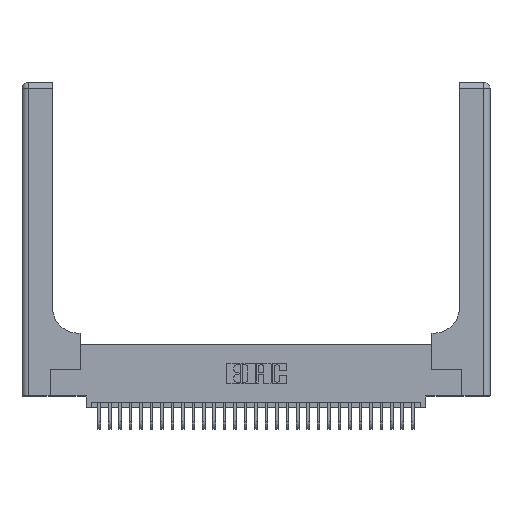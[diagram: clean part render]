
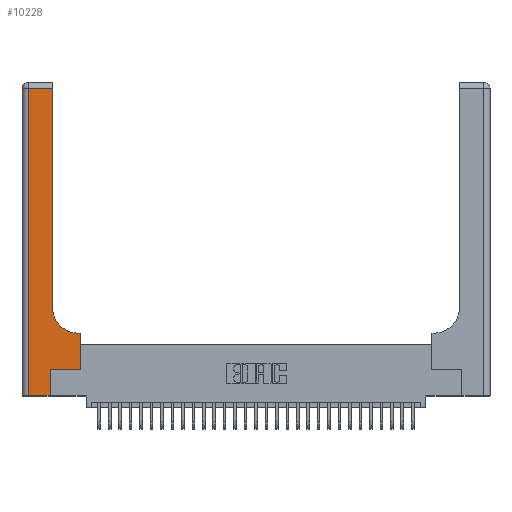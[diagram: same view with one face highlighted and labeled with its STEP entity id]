
A CAD part, top view. The second image highlights one B-rep face of the part: STEP entity #10228.
In plain terms, the highlighted planar face has unit normal (0, 0, 1).
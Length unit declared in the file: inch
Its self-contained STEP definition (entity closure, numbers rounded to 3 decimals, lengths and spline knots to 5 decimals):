
#24 = CARTESIAN_POINT ( 'NONE',  ( 0.2915, 0.85, 0.37 ) ) ;
#1550 = DIRECTION ( 'NONE',  ( 1., 0., 0. ) ) ;
#2169 = VECTOR ( 'NONE', #17892, 39.37008 ) ;
#2900 = LINE ( 'NONE', #7260, #30195 ) ;
#3365 = EDGE_LOOP ( 'NONE', ( #22565, #10003, #14203, #11431, #7960, #29017, #22181, #14543, #21084 ) ) ;
#5346 = EDGE_CURVE ( 'NONE', #19292, #30485, #27529, .T. ) ;
#5491 = CARTESIAN_POINT ( 'NONE',  ( 0.5585, 0.25, 0.37 ) ) ;
#5791 = VECTOR ( 'NONE', #11875, 39.37008 ) ;
#5969 = EDGE_CURVE ( 'NONE', #30485, #29714, #19609, .T. ) ;
#6583 = VERTEX_POINT ( 'NONE', #24 ) ;
#7260 = CARTESIAN_POINT ( 'NONE',  ( 0.269, 0., 0.37 ) ) ;
#7372 = LINE ( 'NONE', #30796, #19226 ) ;
#7460 = EDGE_CURVE ( 'NONE', #29104, #20316, #25124, .T. ) ;
#7960 = ORIENTED_EDGE ( 'NONE', *, *, #15478, .T. ) ;
#8972 = AXIS2_PLACEMENT_3D ( 'NONE', #14369, #19128, #1550 ) ;
#9488 = PLANE ( 'NONE',  #21902 ) ;
#9693 = DIRECTION ( 'NONE',  ( 0., 0., -1. ) ) ;
#9805 = CARTESIAN_POINT ( 'NONE',  ( 0., 3., 0.37 ) ) ;
#10003 = ORIENTED_EDGE ( 'NONE', *, *, #23485, .T. ) ;
#10132 = LINE ( 'NONE', #32572, #5791 ) ;
#10228 = ADVANCED_FACE ( 'NONE', ( #17512 ), #9488, .F. ) ;
#10370 = CARTESIAN_POINT ( 'NONE',  ( 0.5585, 0.25, 0.37 ) ) ;
#10698 = LINE ( 'NONE', #12680, #26083 ) ;
#11087 = CIRCLE ( 'NONE', #8972, 0.25 ) ;
#11431 = ORIENTED_EDGE ( 'NONE', *, *, #5969, .T. ) ;
#11765 = EDGE_CURVE ( 'NONE', #30705, #14472, #10698, .T. ) ;
#11875 = DIRECTION ( 'NONE',  ( 0., 1., 0. ) ) ;
#12680 = CARTESIAN_POINT ( 'NONE',  ( 0.2915, 0.6, 0.37 ) ) ;
#13956 = EDGE_CURVE ( 'NONE', #6583, #17723, #10132, .T. ) ;
#14203 = ORIENTED_EDGE ( 'NONE', *, *, #5346, .T. ) ;
#14369 = CARTESIAN_POINT ( 'NONE',  ( 0.5415, 0.85, 0.37 ) ) ;
#14432 = CARTESIAN_POINT ( 'NONE',  ( 0., 0., 0.37 ) ) ;
#14472 = VERTEX_POINT ( 'NONE', #17046 ) ;
#14543 = ORIENTED_EDGE ( 'NONE', *, *, #11765, .T. ) ;
#15191 = CARTESIAN_POINT ( 'NONE',  ( 0.06, 0., 0.37 ) ) ;
#15478 = EDGE_CURVE ( 'NONE', #29714, #29104, #2900, .T. ) ;
#16627 = CARTESIAN_POINT ( 'NONE',  ( 0.06, 2.94, 0.37 ) ) ;
#16750 = CARTESIAN_POINT ( 'NONE',  ( 0.269, 0.25, 0.37 ) ) ;
#17046 = CARTESIAN_POINT ( 'NONE',  ( 0.5415, 0.6, 0.37 ) ) ;
#17512 = FACE_OUTER_BOUND ( 'NONE', #3365, .T. ) ;
#17723 = VERTEX_POINT ( 'NONE', #25579 ) ;
#17892 = DIRECTION ( 'NONE',  ( 0., 1., 0. ) ) ;
#18237 = CARTESIAN_POINT ( 'NONE',  ( 0.269, 0.25, 0.37 ) ) ;
#19128 = DIRECTION ( 'NONE',  ( 0., 0., -1. ) ) ;
#19226 = VECTOR ( 'NONE', #28451, 39.37008 ) ;
#19292 = VERTEX_POINT ( 'NONE', #16627 ) ;
#19412 = DIRECTION ( 'NONE',  ( 1., 0., 0. ) ) ;
#19482 = DIRECTION ( 'NONE',  ( 1., 0., 0. ) ) ;
#19609 = LINE ( 'NONE', #14432, #29088 ) ;
#19666 = CARTESIAN_POINT ( 'NONE',  ( 0.269, 0., 0.37 ) ) ;
#20316 = VERTEX_POINT ( 'NONE', #5491 ) ;
#21084 = ORIENTED_EDGE ( 'NONE', *, *, #29605, .T. ) ;
#21213 = VECTOR ( 'NONE', #19482, 39.37008 ) ;
#21902 = AXIS2_PLACEMENT_3D ( 'NONE', #9805, #9693, #22364 ) ;
#22181 = ORIENTED_EDGE ( 'NONE', *, *, #25624, .T. ) ;
#22353 = DIRECTION ( 'NONE',  ( 0., 1., 0. ) ) ;
#22364 = DIRECTION ( 'NONE',  ( -1., 0., 0. ) ) ;
#22565 = ORIENTED_EDGE ( 'NONE', *, *, #13956, .T. ) ;
#23113 = DIRECTION ( 'NONE',  ( -1., 0., 0. ) ) ;
#23485 = EDGE_CURVE ( 'NONE', #17723, #19292, #7372, .T. ) ;
#23487 = LINE ( 'NONE', #10370, #2169 ) ;
#23992 = VECTOR ( 'NONE', #24066, 39.37008 ) ;
#24066 = DIRECTION ( 'NONE',  ( 0., -1., 0. ) ) ;
#24393 = CARTESIAN_POINT ( 'NONE',  ( 0.06, 3., 0.37 ) ) ;
#25124 = LINE ( 'NONE', #18237, #21213 ) ;
#25579 = CARTESIAN_POINT ( 'NONE',  ( 0.2915, 2.94, 0.37 ) ) ;
#25624 = EDGE_CURVE ( 'NONE', #20316, #30705, #23487, .T. ) ;
#26083 = VECTOR ( 'NONE', #23113, 39.37008 ) ;
#27529 = LINE ( 'NONE', #24393, #23992 ) ;
#28451 = DIRECTION ( 'NONE',  ( -1., 0., 0. ) ) ;
#29017 = ORIENTED_EDGE ( 'NONE', *, *, #7460, .T. ) ;
#29088 = VECTOR ( 'NONE', #19412, 39.37008 ) ;
#29104 = VERTEX_POINT ( 'NONE', #16750 ) ;
#29605 = EDGE_CURVE ( 'NONE', #14472, #6583, #11087, .T. ) ;
#29714 = VERTEX_POINT ( 'NONE', #19666 ) ;
#30195 = VECTOR ( 'NONE', #22353, 39.37008 ) ;
#30485 = VERTEX_POINT ( 'NONE', #15191 ) ;
#30705 = VERTEX_POINT ( 'NONE', #30775 ) ;
#30775 = CARTESIAN_POINT ( 'NONE',  ( 0.5585, 0.6, 0.37 ) ) ;
#30796 = CARTESIAN_POINT ( 'NONE',  ( 0., 2.94, 0.37 ) ) ;
#32572 = CARTESIAN_POINT ( 'NONE',  ( 0.2915, 3., 0.37 ) ) ;
